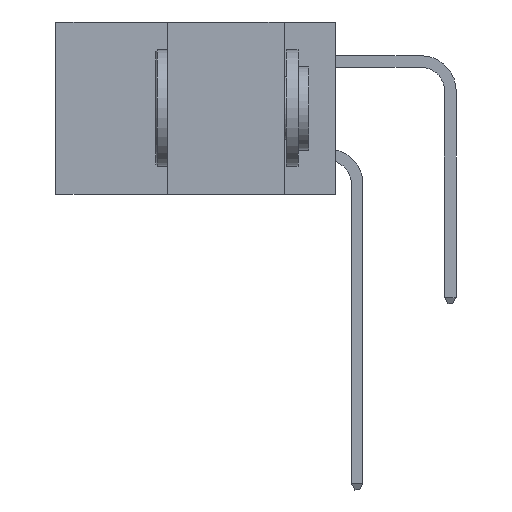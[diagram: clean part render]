
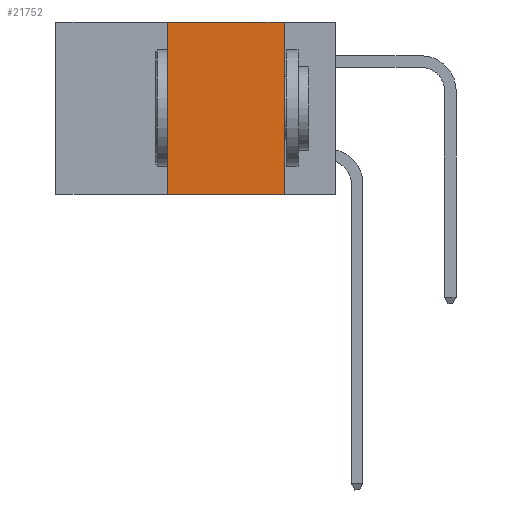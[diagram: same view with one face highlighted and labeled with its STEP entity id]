
A CAD part, left-side view. The second image highlights one B-rep face of the part: STEP entity #21752.
In plain terms, the highlighted planar face has unit normal (-1, 0, 0).
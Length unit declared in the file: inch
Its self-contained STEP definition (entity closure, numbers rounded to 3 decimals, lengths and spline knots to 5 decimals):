
#805 = EDGE_LOOP ( 'NONE', ( #11822, #20928, #6498, #23638 ) ) ;
#2102 = FACE_OUTER_BOUND ( 'NONE', #805, .T. ) ;
#3383 = CARTESIAN_POINT ( 'NONE',  ( 0., 0.6, 0. ) ) ;
#5681 = VECTOR ( 'NONE', #7141, 39.37008 ) ;
#6290 = DIRECTION ( 'NONE',  ( 0., 0., -1. ) ) ;
#6498 = ORIENTED_EDGE ( 'NONE', *, *, #13993, .F. ) ;
#7141 = DIRECTION ( 'NONE',  ( 0., 0., -1. ) ) ;
#8457 = LINE ( 'NONE', #12598, #29913 ) ;
#9188 = CARTESIAN_POINT ( 'NONE',  ( 0., 0.36, 0. ) ) ;
#9355 = EDGE_CURVE ( 'NONE', #12591, #19247, #17007, .T. ) ;
#10210 = EDGE_CURVE ( 'NONE', #15826, #12591, #8457, .T. ) ;
#10387 = DIRECTION ( 'NONE',  ( 0., -1., 0. ) ) ;
#11822 = ORIENTED_EDGE ( 'NONE', *, *, #9355, .F. ) ;
#12591 = VERTEX_POINT ( 'NONE', #25173 ) ;
#12598 = CARTESIAN_POINT ( 'NONE',  ( 0., 0.6, 0. ) ) ;
#13993 = EDGE_CURVE ( 'NONE', #14231, #15826, #17178, .T. ) ;
#14231 = VERTEX_POINT ( 'NONE', #21310 ) ;
#14737 = CARTESIAN_POINT ( 'NONE',  ( 0., 0.11, 0. ) ) ;
#15826 = VERTEX_POINT ( 'NONE', #22482 ) ;
#16578 = DIRECTION ( 'NONE',  ( 1., 0., 0. ) ) ;
#17007 = LINE ( 'NONE', #14737, #5681 ) ;
#17178 = LINE ( 'NONE', #9188, #24043 ) ;
#19247 = VERTEX_POINT ( 'NONE', #21383 ) ;
#20260 = DIRECTION ( 'NONE',  ( 0., -1., 0. ) ) ;
#20668 = CARTESIAN_POINT ( 'NONE',  ( 0., 0.6, -0.37 ) ) ;
#20928 = ORIENTED_EDGE ( 'NONE', *, *, #10210, .F. ) ;
#21272 = LINE ( 'NONE', #20668, #27794 ) ;
#21310 = CARTESIAN_POINT ( 'NONE',  ( 0., 0.36, -0.37 ) ) ;
#21383 = CARTESIAN_POINT ( 'NONE',  ( 0., 0.11, -0.37 ) ) ;
#21752 = ADVANCED_FACE ( 'NONE', ( #2102 ), #32062, .F. ) ;
#22482 = CARTESIAN_POINT ( 'NONE',  ( 0., 0.36, 0. ) ) ;
#23638 = ORIENTED_EDGE ( 'NONE', *, *, #32489, .T. ) ;
#24043 = VECTOR ( 'NONE', #30210, 39.37008 ) ;
#25173 = CARTESIAN_POINT ( 'NONE',  ( 0., 0.11, 0. ) ) ;
#27794 = VECTOR ( 'NONE', #10387, 39.37008 ) ;
#29913 = VECTOR ( 'NONE', #20260, 39.37008 ) ;
#30210 = DIRECTION ( 'NONE',  ( 0., 0., 1. ) ) ;
#30532 = AXIS2_PLACEMENT_3D ( 'NONE', #3383, #16578, #6290 ) ;
#32062 = PLANE ( 'NONE',  #30532 ) ;
#32489 = EDGE_CURVE ( 'NONE', #14231, #19247, #21272, .T. ) ;
